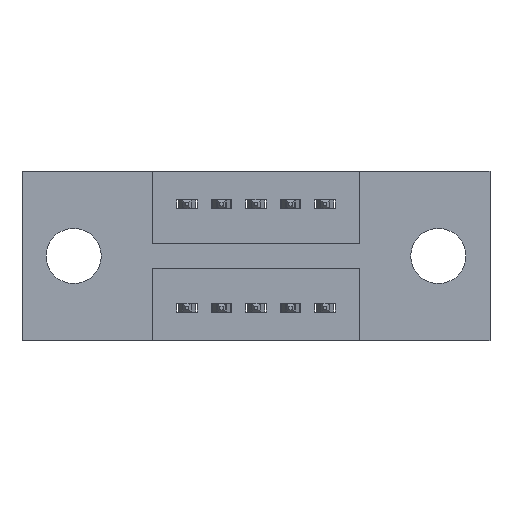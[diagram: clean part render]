
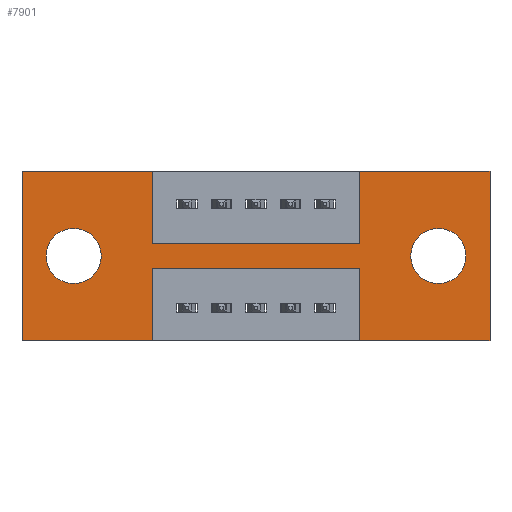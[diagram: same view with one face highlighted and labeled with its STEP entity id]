
A CAD part, front view. The second image highlights one B-rep face of the part: STEP entity #7901.
In plain terms, the highlighted planar face has unit normal (0, -1, 0).
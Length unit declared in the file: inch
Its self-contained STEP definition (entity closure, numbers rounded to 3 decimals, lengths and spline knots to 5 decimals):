
#146 = EDGE_CURVE ( 'NONE', #1972, #6915, #3716, .T. ) ;
#167 = CARTESIAN_POINT ( 'NONE',  ( 0.3775, 0., -0.28 ) ) ;
#205 = DIRECTION ( 'NONE',  ( 0., 0., -1. ) ) ;
#257 = ORIENTED_EDGE ( 'NONE', *, *, #980, .F. ) ;
#273 = CARTESIAN_POINT ( 'NONE',  ( 1.2055, 0., -0.325 ) ) ;
#282 = EDGE_CURVE ( 'NONE', #7798, #2425, #4086, .T. ) ;
#300 = EDGE_CURVE ( 'NONE', #2425, #5942, #7407, .T. ) ;
#305 = DIRECTION ( 'NONE',  ( -1., 0., 0. ) ) ;
#323 = CARTESIAN_POINT ( 'NONE',  ( 0., 0., 0. ) ) ;
#332 = CARTESIAN_POINT ( 'NONE',  ( 0., 0., -0.49 ) ) ;
#414 = ORIENTED_EDGE ( 'NONE', *, *, #4000, .F. ) ;
#433 = VERTEX_POINT ( 'NONE', #3354 ) ;
#446 = CARTESIAN_POINT ( 'NONE',  ( 0.1495, 0., -0.325 ) ) ;
#470 = DIRECTION ( 'NONE',  ( 0., 1., 0. ) ) ;
#517 = ORIENTED_EDGE ( 'NONE', *, *, #5927, .F. ) ;
#526 = CARTESIAN_POINT ( 'NONE',  ( 0.9775, 0., -0.49 ) ) ;
#559 = ORIENTED_EDGE ( 'NONE', *, *, #3507, .F. ) ;
#644 = VERTEX_POINT ( 'NONE', #7337 ) ;
#649 = VECTOR ( 'NONE', #205, 39.37008 ) ;
#668 = EDGE_CURVE ( 'NONE', #7418, #7340, #2356, .T. ) ;
#773 = LINE ( 'NONE', #6468, #3375 ) ;
#866 = ORIENTED_EDGE ( 'NONE', *, *, #3871, .F. ) ;
#876 = ORIENTED_EDGE ( 'NONE', *, *, #282, .F. ) ;
#953 = VERTEX_POINT ( 'NONE', #1871 ) ;
#955 = DIRECTION ( 'NONE',  ( 1., 0., 0. ) ) ;
#980 = EDGE_CURVE ( 'NONE', #6915, #3624, #2157, .T. ) ;
#1005 = ORIENTED_EDGE ( 'NONE', *, *, #668, .T. ) ;
#1053 = EDGE_CURVE ( 'NONE', #5942, #953, #1491, .T. ) ;
#1094 = DIRECTION ( 'NONE',  ( 0., 0., -1. ) ) ;
#1177 = CIRCLE ( 'NONE', #7132, 0.08 ) ;
#1226 = DIRECTION ( 'NONE',  ( 0., -1., 0. ) ) ;
#1491 = LINE ( 'NONE', #167, #6006 ) ;
#1717 = EDGE_CURVE ( 'NONE', #7340, #7418, #2831, .T. ) ;
#1812 = CARTESIAN_POINT ( 'NONE',  ( 0., 0., -0.49 ) ) ;
#1837 = ORIENTED_EDGE ( 'NONE', *, *, #6615, .F. ) ;
#1871 = CARTESIAN_POINT ( 'NONE',  ( 0.3775, 0., -0.28 ) ) ;
#1930 = VECTOR ( 'NONE', #5960, 39.37008 ) ;
#1966 = CARTESIAN_POINT ( 'NONE',  ( 1.355, 0., -0.49 ) ) ;
#1972 = VERTEX_POINT ( 'NONE', #3241 ) ;
#1992 = EDGE_LOOP ( 'NONE', ( #4498, #4385 ) ) ;
#2026 = DIRECTION ( 'NONE',  ( -1., 0., 0. ) ) ;
#2027 = CARTESIAN_POINT ( 'NONE',  ( 1.355, 0., 0. ) ) ;
#2034 = FACE_BOUND ( 'NONE', #1992, .T. ) ;
#2060 = LINE ( 'NONE', #5598, #6004 ) ;
#2147 = CARTESIAN_POINT ( 'NONE',  ( 0., 0., 0. ) ) ;
#2157 = LINE ( 'NONE', #5533, #6101 ) ;
#2258 = VECTOR ( 'NONE', #305, 39.37008 ) ;
#2356 = CIRCLE ( 'NONE', #3669, 0.08 ) ;
#2425 = VERTEX_POINT ( 'NONE', #526 ) ;
#2456 = EDGE_CURVE ( 'NONE', #5696, #4783, #1177, .T. ) ;
#2656 = LINE ( 'NONE', #5163, #7604 ) ;
#2693 = CARTESIAN_POINT ( 'NONE',  ( 0.9775, 0., -0.28 ) ) ;
#2770 = LINE ( 'NONE', #3069, #3528 ) ;
#2831 = CIRCLE ( 'NONE', #5160, 0.08 ) ;
#2862 = DIRECTION ( 'NONE',  ( 0., 0., 1. ) ) ;
#2997 = LINE ( 'NONE', #323, #5957 ) ;
#3065 = DIRECTION ( 'NONE',  ( 0., 1., 0. ) ) ;
#3069 = CARTESIAN_POINT ( 'NONE',  ( 0.3775, 0., -0.28 ) ) ;
#3099 = CIRCLE ( 'NONE', #3884, 0.08 ) ;
#3215 = PLANE ( 'NONE',  #5362 ) ;
#3241 = CARTESIAN_POINT ( 'NONE',  ( 0.3775, 0., 0. ) ) ;
#3263 = ORIENTED_EDGE ( 'NONE', *, *, #300, .F. ) ;
#3354 = CARTESIAN_POINT ( 'NONE',  ( 0., 0., 0. ) ) ;
#3370 = CARTESIAN_POINT ( 'NONE',  ( 0.9775, 0., -0.28 ) ) ;
#3375 = VECTOR ( 'NONE', #5919, 39.37008 ) ;
#3507 = EDGE_CURVE ( 'NONE', #6914, #7798, #773, .T. ) ;
#3528 = VECTOR ( 'NONE', #7956, 39.37008 ) ;
#3564 = LINE ( 'NONE', #2147, #1930 ) ;
#3624 = VERTEX_POINT ( 'NONE', #4735 ) ;
#3626 = CARTESIAN_POINT ( 'NONE',  ( 0.1495, 0., -0.245 ) ) ;
#3627 = CARTESIAN_POINT ( 'NONE',  ( 0.9775, 0., 0. ) ) ;
#3635 = DIRECTION ( 'NONE',  ( -1., 0., 0. ) ) ;
#3669 = AXIS2_PLACEMENT_3D ( 'NONE', #3626, #7495, #7467 ) ;
#3716 = LINE ( 'NONE', #6314, #649 ) ;
#3740 = EDGE_CURVE ( 'NONE', #433, #1972, #3564, .T. ) ;
#3871 = EDGE_CURVE ( 'NONE', #5216, #6914, #2997, .T. ) ;
#3884 = AXIS2_PLACEMENT_3D ( 'NONE', #4139, #7834, #7444 ) ;
#4000 = EDGE_CURVE ( 'NONE', #6277, #644, #5078, .T. ) ;
#4086 = LINE ( 'NONE', #332, #2258 ) ;
#4139 = CARTESIAN_POINT ( 'NONE',  ( 1.2055, 0., -0.245 ) ) ;
#4385 = ORIENTED_EDGE ( 'NONE', *, *, #7986, .T. ) ;
#4498 = ORIENTED_EDGE ( 'NONE', *, *, #2456, .T. ) ;
#4571 = ORIENTED_EDGE ( 'NONE', *, *, #1053, .F. ) ;
#4641 = ORIENTED_EDGE ( 'NONE', *, *, #3740, .F. ) ;
#4709 = FACE_OUTER_BOUND ( 'NONE', #6866, .T. ) ;
#4735 = CARTESIAN_POINT ( 'NONE',  ( 0.9775, 0., -0.21 ) ) ;
#4783 = VERTEX_POINT ( 'NONE', #273 ) ;
#4946 = CARTESIAN_POINT ( 'NONE',  ( 0.1495, 0., -0.245 ) ) ;
#5053 = ORIENTED_EDGE ( 'NONE', *, *, #5294, .F. ) ;
#5078 = LINE ( 'NONE', #5450, #5864 ) ;
#5160 = AXIS2_PLACEMENT_3D ( 'NONE', #4946, #3065, #8032 ) ;
#5163 = CARTESIAN_POINT ( 'NONE',  ( 0., 0., 0. ) ) ;
#5216 = VERTEX_POINT ( 'NONE', #3627 ) ;
#5294 = EDGE_CURVE ( 'NONE', #953, #6277, #2770, .T. ) ;
#5362 = AXIS2_PLACEMENT_3D ( 'NONE', #1812, #1226, #5428 ) ;
#5428 = DIRECTION ( 'NONE',  ( 0., 0., -1. ) ) ;
#5450 = CARTESIAN_POINT ( 'NONE',  ( 0., 0., -0.49 ) ) ;
#5533 = CARTESIAN_POINT ( 'NONE',  ( 0.3775, 0., -0.21 ) ) ;
#5598 = CARTESIAN_POINT ( 'NONE',  ( 0.9775, 0., -0.21 ) ) ;
#5696 = VERTEX_POINT ( 'NONE', #6562 ) ;
#5864 = VECTOR ( 'NONE', #3635, 39.37008 ) ;
#5919 = DIRECTION ( 'NONE',  ( 0., 0., -1. ) ) ;
#5927 = EDGE_CURVE ( 'NONE', #644, #433, #2656, .T. ) ;
#5942 = VERTEX_POINT ( 'NONE', #2693 ) ;
#5957 = VECTOR ( 'NONE', #955, 39.37008 ) ;
#5960 = DIRECTION ( 'NONE',  ( 1., 0., 0. ) ) ;
#5981 = FACE_BOUND ( 'NONE', #6506, .T. ) ;
#6004 = VECTOR ( 'NONE', #2862, 39.37008 ) ;
#6006 = VECTOR ( 'NONE', #2026, 39.37008 ) ;
#6019 = ORIENTED_EDGE ( 'NONE', *, *, #146, .F. ) ;
#6101 = VECTOR ( 'NONE', #6836, 39.37008 ) ;
#6277 = VERTEX_POINT ( 'NONE', #7455 ) ;
#6314 = CARTESIAN_POINT ( 'NONE',  ( 0.3775, 0., -0.21 ) ) ;
#6468 = CARTESIAN_POINT ( 'NONE',  ( 1.355, 0., 0. ) ) ;
#6506 = EDGE_LOOP ( 'NONE', ( #7632, #1005 ) ) ;
#6562 = CARTESIAN_POINT ( 'NONE',  ( 1.2055, 0., -0.165 ) ) ;
#6615 = EDGE_CURVE ( 'NONE', #3624, #5216, #2060, .T. ) ;
#6836 = DIRECTION ( 'NONE',  ( 1., 0., 0. ) ) ;
#6866 = EDGE_LOOP ( 'NONE', ( #1837, #257, #6019, #4641, #517, #414, #5053, #4571, #3263, #876, #559, #866 ) ) ;
#6914 = VERTEX_POINT ( 'NONE', #2027 ) ;
#6915 = VERTEX_POINT ( 'NONE', #7751 ) ;
#7132 = AXIS2_PLACEMENT_3D ( 'NONE', #7290, #470, #1094 ) ;
#7290 = CARTESIAN_POINT ( 'NONE',  ( 1.2055, 0., -0.245 ) ) ;
#7337 = CARTESIAN_POINT ( 'NONE',  ( 0., 0., -0.49 ) ) ;
#7340 = VERTEX_POINT ( 'NONE', #7814 ) ;
#7407 = LINE ( 'NONE', #3370, #7893 ) ;
#7418 = VERTEX_POINT ( 'NONE', #446 ) ;
#7444 = DIRECTION ( 'NONE',  ( 0., 0., -1. ) ) ;
#7455 = CARTESIAN_POINT ( 'NONE',  ( 0.3775, 0., -0.49 ) ) ;
#7467 = DIRECTION ( 'NONE',  ( 0., 0., 1. ) ) ;
#7495 = DIRECTION ( 'NONE',  ( 0., 1., 0. ) ) ;
#7599 = DIRECTION ( 'NONE',  ( 0., 0., 1. ) ) ;
#7604 = VECTOR ( 'NONE', #7599, 39.37008 ) ;
#7632 = ORIENTED_EDGE ( 'NONE', *, *, #1717, .T. ) ;
#7751 = CARTESIAN_POINT ( 'NONE',  ( 0.3775, 0., -0.21 ) ) ;
#7756 = DIRECTION ( 'NONE',  ( 0., 0., 1. ) ) ;
#7798 = VERTEX_POINT ( 'NONE', #1966 ) ;
#7814 = CARTESIAN_POINT ( 'NONE',  ( 0.1495, 0., -0.165 ) ) ;
#7834 = DIRECTION ( 'NONE',  ( 0., 1., 0. ) ) ;
#7893 = VECTOR ( 'NONE', #7756, 39.37008 ) ;
#7901 = ADVANCED_FACE ( 'NONE', ( #2034, #5981, #4709 ), #3215, .T. ) ;
#7956 = DIRECTION ( 'NONE',  ( 0., 0., -1. ) ) ;
#7986 = EDGE_CURVE ( 'NONE', #4783, #5696, #3099, .T. ) ;
#8032 = DIRECTION ( 'NONE',  ( 0., 0., 1. ) ) ;
